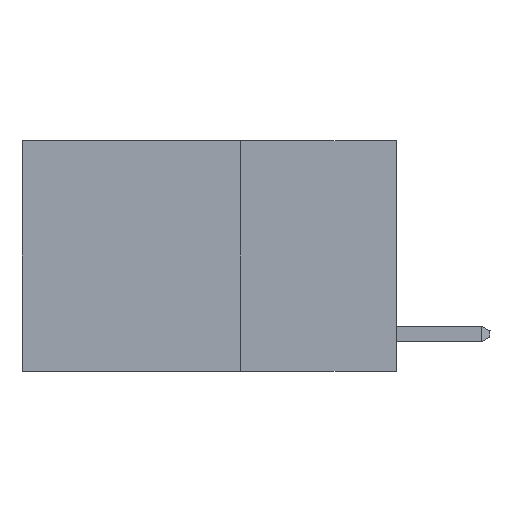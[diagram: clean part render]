
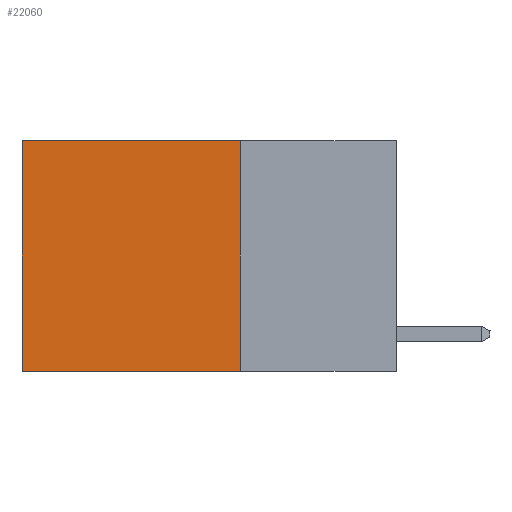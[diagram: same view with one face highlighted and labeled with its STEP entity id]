
A CAD part, left-side view. The second image highlights one B-rep face of the part: STEP entity #22060.
In plain terms, the highlighted planar face has unit normal (-1, 0, 0).
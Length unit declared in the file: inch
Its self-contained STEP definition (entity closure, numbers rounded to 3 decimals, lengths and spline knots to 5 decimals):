
#719 = ORIENTED_EDGE ( 'NONE', *, *, #15142, .T. ) ;
#827 = CARTESIAN_POINT ( 'NONE',  ( 0.2625, 0.25, 0. ) ) ;
#1535 = CARTESIAN_POINT ( 'NONE',  ( 0.2625, 0.6, 0. ) ) ;
#2116 = VECTOR ( 'NONE', #27207, 39.37008 ) ;
#2246 = VERTEX_POINT ( 'NONE', #25708 ) ;
#5472 = ORIENTED_EDGE ( 'NONE', *, *, #16396, .F. ) ;
#5651 = CARTESIAN_POINT ( 'NONE',  ( 0.2625, 0.6, 0. ) ) ;
#6159 = DIRECTION ( 'NONE',  ( 1., 0., 0. ) ) ;
#6866 = EDGE_CURVE ( 'NONE', #23498, #20576, #25497, .T. ) ;
#8808 = VECTOR ( 'NONE', #27091, 39.37008 ) ;
#9594 = VERTEX_POINT ( 'NONE', #17065 ) ;
#10495 = CARTESIAN_POINT ( 'NONE',  ( 0.2625, 0.25, 0. ) ) ;
#11064 = DIRECTION ( 'NONE',  ( 0., 0., -1. ) ) ;
#11834 = CARTESIAN_POINT ( 'NONE',  ( 0.2625, 0.25, -0.37 ) ) ;
#12067 = EDGE_CURVE ( 'NONE', #23498, #2246, #23778, .T. ) ;
#12212 = ORIENTED_EDGE ( 'NONE', *, *, #12067, .F. ) ;
#13220 = FACE_OUTER_BOUND ( 'NONE', #17774, .T. ) ;
#15142 = EDGE_CURVE ( 'NONE', #20576, #9594, #26824, .T. ) ;
#16321 = DIRECTION ( 'NONE',  ( 0., 1., 0. ) ) ;
#16396 = EDGE_CURVE ( 'NONE', #2246, #9594, #27099, .T. ) ;
#17065 = CARTESIAN_POINT ( 'NONE',  ( 0.2625, 0.6, -0.37 ) ) ;
#17292 = PLANE ( 'NONE',  #22824 ) ;
#17774 = EDGE_LOOP ( 'NONE', ( #719, #5472, #12212, #22934 ) ) ;
#20576 = VERTEX_POINT ( 'NONE', #5651 ) ;
#22060 = ADVANCED_FACE ( 'NONE', ( #13220 ), #17292, .F. ) ;
#22824 = AXIS2_PLACEMENT_3D ( 'NONE', #10495, #6159, #23783 ) ;
#22934 = ORIENTED_EDGE ( 'NONE', *, *, #6866, .T. ) ;
#23498 = VERTEX_POINT ( 'NONE', #24918 ) ;
#23778 = LINE ( 'NONE', #28345, #24409 ) ;
#23783 = DIRECTION ( 'NONE',  ( 0., 0., -1. ) ) ;
#24409 = VECTOR ( 'NONE', #11064, 39.37008 ) ;
#24918 = CARTESIAN_POINT ( 'NONE',  ( 0.2625, 0.25, 0. ) ) ;
#25497 = LINE ( 'NONE', #827, #2116 ) ;
#25708 = CARTESIAN_POINT ( 'NONE',  ( 0.2625, 0.25, -0.37 ) ) ;
#26787 = VECTOR ( 'NONE', #16321, 39.37008 ) ;
#26824 = LINE ( 'NONE', #1535, #8808 ) ;
#27091 = DIRECTION ( 'NONE',  ( 0., 0., -1. ) ) ;
#27099 = LINE ( 'NONE', #11834, #26787 ) ;
#27207 = DIRECTION ( 'NONE',  ( 0., 1., 0. ) ) ;
#28345 = CARTESIAN_POINT ( 'NONE',  ( 0.2625, 0.25, 0. ) ) ;
